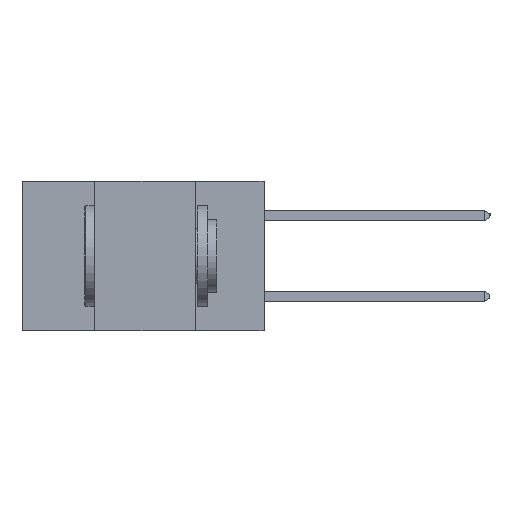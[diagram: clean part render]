
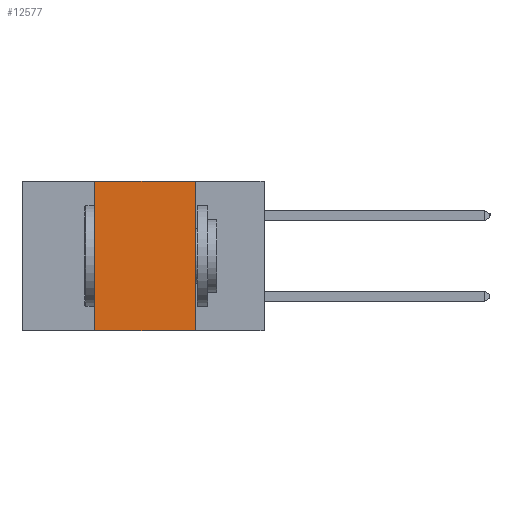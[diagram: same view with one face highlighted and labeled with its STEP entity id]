
A CAD part, left-side view. The second image highlights one B-rep face of the part: STEP entity #12577.
In plain terms, the highlighted planar face has unit normal (-1, 0, 0).
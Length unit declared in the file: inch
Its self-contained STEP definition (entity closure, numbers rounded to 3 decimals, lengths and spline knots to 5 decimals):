
#111 = CARTESIAN_POINT ( 'NONE',  ( 0., 0.6, 0. ) ) ;
#1017 = CARTESIAN_POINT ( 'NONE',  ( 0., 0.6, -0.37 ) ) ;
#1093 = FACE_OUTER_BOUND ( 'NONE', #8811, .T. ) ;
#1135 = VERTEX_POINT ( 'NONE', #7995 ) ;
#1227 = LINE ( 'NONE', #1017, #9520 ) ;
#1285 = AXIS2_PLACEMENT_3D ( 'NONE', #111, #3298, #9652 ) ;
#1295 = LINE ( 'NONE', #10579, #5662 ) ;
#1324 = CARTESIAN_POINT ( 'NONE',  ( 0., 0.17, 0. ) ) ;
#1634 = EDGE_CURVE ( 'NONE', #5938, #1135, #1824, .T. ) ;
#1824 = LINE ( 'NONE', #1958, #6798 ) ;
#1958 = CARTESIAN_POINT ( 'NONE',  ( 0., 0.17, -0.37 ) ) ;
#2239 = EDGE_CURVE ( 'NONE', #8330, #1135, #1227, .T. ) ;
#2275 = ORIENTED_EDGE ( 'NONE', *, *, #2239, .T. ) ;
#3298 = DIRECTION ( 'NONE',  ( 1., 0., 0. ) ) ;
#4767 = CARTESIAN_POINT ( 'NONE',  ( 0., 0.42, -0.37 ) ) ;
#5159 = DIRECTION ( 'NONE',  ( 0., 0., -1. ) ) ;
#5251 = DIRECTION ( 'NONE',  ( 0., -1., 0. ) ) ;
#5662 = VECTOR ( 'NONE', #13761, 39.37008 ) ;
#5938 = VERTEX_POINT ( 'NONE', #1324 ) ;
#6145 = EDGE_CURVE ( 'NONE', #8330, #6403, #1295, .T. ) ;
#6403 = VERTEX_POINT ( 'NONE', #7991 ) ;
#6559 = EDGE_CURVE ( 'NONE', #6403, #5938, #12615, .T. ) ;
#6798 = VECTOR ( 'NONE', #5159, 39.37008 ) ;
#7472 = ORIENTED_EDGE ( 'NONE', *, *, #1634, .F. ) ;
#7991 = CARTESIAN_POINT ( 'NONE',  ( 0., 0.42, 0. ) ) ;
#7995 = CARTESIAN_POINT ( 'NONE',  ( 0., 0.17, -0.37 ) ) ;
#8279 = ORIENTED_EDGE ( 'NONE', *, *, #6145, .F. ) ;
#8330 = VERTEX_POINT ( 'NONE', #4767 ) ;
#8570 = PLANE ( 'NONE',  #1285 ) ;
#8811 = EDGE_LOOP ( 'NONE', ( #7472, #10213, #8279, #2275 ) ) ;
#9520 = VECTOR ( 'NONE', #10639, 39.37008 ) ;
#9652 = DIRECTION ( 'NONE',  ( 0., 0., -1. ) ) ;
#10213 = ORIENTED_EDGE ( 'NONE', *, *, #6559, .F. ) ;
#10345 = CARTESIAN_POINT ( 'NONE',  ( 0., 0.6, 0. ) ) ;
#10579 = CARTESIAN_POINT ( 'NONE',  ( 0., 0.42, -0.37 ) ) ;
#10639 = DIRECTION ( 'NONE',  ( 0., -1., 0. ) ) ;
#10899 = VECTOR ( 'NONE', #5251, 39.37008 ) ;
#12577 = ADVANCED_FACE ( 'NONE', ( #1093 ), #8570, .F. ) ;
#12615 = LINE ( 'NONE', #10345, #10899 ) ;
#13761 = DIRECTION ( 'NONE',  ( 0., 0., 1. ) ) ;
